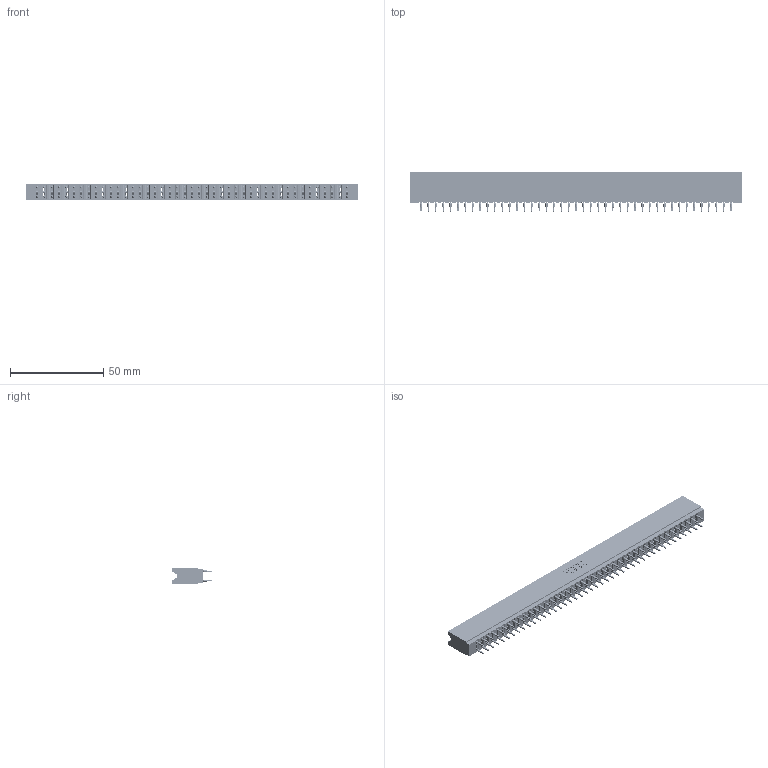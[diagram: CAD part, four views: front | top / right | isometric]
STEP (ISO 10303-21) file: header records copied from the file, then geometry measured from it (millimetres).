
FILE_DESCRIPTION (( 'STEP AP203' ), '1' );
FILE_NAME ('737-086-560-206.STEP', '2026-03-06T02:37:27', ( '' ), ( '' ), 'SwSTEP 2.0', 'SolidWorks 2023', '' );
FILE_SCHEMA (( 'CONFIG_CONTROL_DESIGN' ));
Length unit declared in the file: millimetre
Products named in the file (3): 745-292-001_560; 737-086-560-206; 737 Part_Insulator Option - 06
Assembly tree (87 placements, depth 2):
  737-086-560-206
    737 Part_Insulator Option - 06
    745-292-001_560  x86
Bounding box: 178.26 x 21.22 x 8.89 mm (x, y, z)
Volume: 17848.8 mm3; surface area: 27865.5 mm2
Topology: 87 solids, 87 shells, 8609 faces, 23563 edges, 14962 vertices
Faces by surface type: plane 4484, cylinder 1889, bspline 1720, torus 516
Entity records: 73984 total; most frequent: CARTESIAN_POINT 13348, ORIENTED_EDGE 12786, DIRECTION 11163, EDGE_CURVE 6393, LINE 5945, VECTOR 5945, VERTEX_POINT 4082, AXIS2_PLACEMENT_3D 2609
